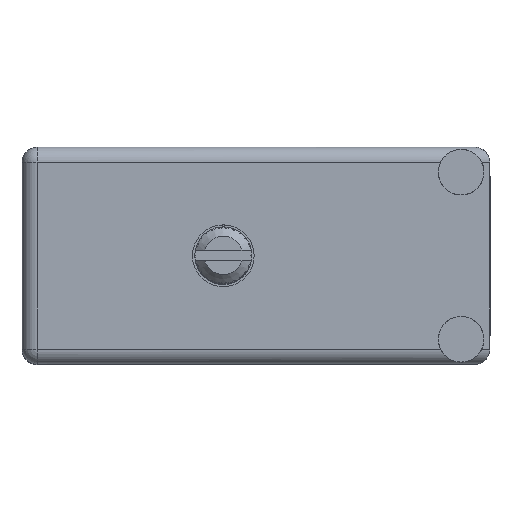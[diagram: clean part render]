
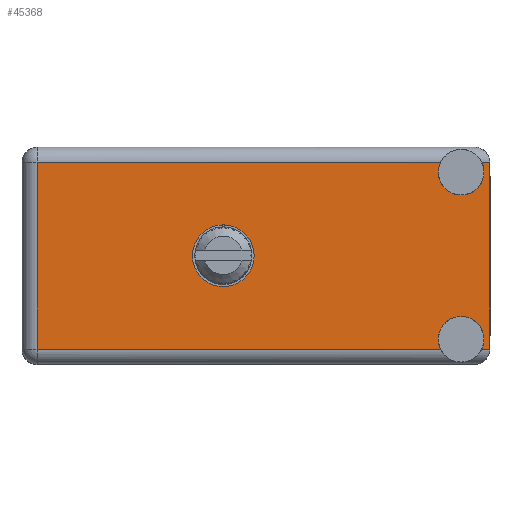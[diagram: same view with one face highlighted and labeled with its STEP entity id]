
A CAD part, top view. The second image highlights one B-rep face of the part: STEP entity #45368.
In plain terms, the highlighted face is planar.
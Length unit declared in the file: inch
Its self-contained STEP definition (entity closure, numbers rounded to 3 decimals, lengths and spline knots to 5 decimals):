
#1294 = VERTEX_POINT ( 'NONE', #162878 ) ;
#2491 = LINE ( 'NONE', #105582, #120860 ) ;
#3079 = EDGE_CURVE ( 'NONE', #1294, #177428, #159505, .T. ) ;
#6023 = ORIENTED_EDGE ( 'NONE', *, *, #139599, .F. ) ;
#8165 = EDGE_LOOP ( 'NONE', ( #48326, #6023, #74118, #162104, #158377, #182573, #144816, #176482, #103354, #86603 ) ) ;
#10953 = CARTESIAN_POINT ( 'NONE',  ( 1.445, 0.906, -0.1575 ) ) ;
#11195 = AXIS2_PLACEMENT_3D ( 'NONE', #15389, #90381, #115714 ) ;
#13502 = ORIENTED_EDGE ( 'NONE', *, *, #179214, .F. ) ;
#15389 = CARTESIAN_POINT ( 'NONE',  ( 1.445, 0.906, -0.6325 ) ) ;
#28520 = DIRECTION ( 'NONE',  ( 0., 0., 1. ) ) ;
#30066 = DIRECTION ( 'NONE',  ( -1., 0., 0. ) ) ;
#32092 = LINE ( 'NONE', #105170, #139621 ) ;
#32625 = DIRECTION ( 'NONE',  ( 1., 0., 0. ) ) ;
#34725 = VECTOR ( 'NONE', #75113, 39.37008 ) ;
#34835 = DIRECTION ( 'NONE',  ( 1., 0., 0. ) ) ;
#39893 = EDGE_CURVE ( 'NONE', #51134, #92540, #2491, .T. ) ;
#41580 = CIRCLE ( 'NONE', #113403, 0.075 ) ;
#43859 = DIRECTION ( 'NONE',  ( 0., 0., 1. ) ) ;
#45368 = ADVANCED_FACE ( 'NONE', ( #126077, #184150 ), #56694, .T. ) ;
#46123 = CARTESIAN_POINT ( 'NONE',  ( 1.445, 0.906, -0.0825 ) ) ;
#47203 = CIRCLE ( 'NONE', #163909, 0.1015 ) ;
#47387 = CARTESIAN_POINT ( 'NONE',  ( 0.6625, 0.906, -0.3575 ) ) ;
#47445 = ORIENTED_EDGE ( 'NONE', *, *, #75658, .F. ) ;
#48018 = DIRECTION ( 'NONE',  ( 0., 0., 1. ) ) ;
#48326 = ORIENTED_EDGE ( 'NONE', *, *, #91552, .T. ) ;
#49850 = DIRECTION ( 'NONE',  ( -1., 0., 0. ) ) ;
#49929 = CIRCLE ( 'NONE', #175555, 0.1015 ) ;
#51134 = VERTEX_POINT ( 'NONE', #149179 ) ;
#51189 = VERTEX_POINT ( 'NONE', #95678 ) ;
#56694 = PLANE ( 'NONE',  #162783 ) ;
#59122 = VERTEX_POINT ( 'NONE', #104556 ) ;
#59716 = DIRECTION ( 'NONE',  ( 0., 0., 1. ) ) ;
#60957 = CARTESIAN_POINT ( 'NONE',  ( 1.539, 0.906, -0.05 ) ) ;
#73524 = DIRECTION ( 'NONE',  ( 0., 0., 1. ) ) ;
#74118 = ORIENTED_EDGE ( 'NONE', *, *, #185371, .F. ) ;
#74225 = VERTEX_POINT ( 'NONE', #184911 ) ;
#74305 = EDGE_CURVE ( 'NONE', #51134, #59122, #32092, .T. ) ;
#75113 = DIRECTION ( 'NONE',  ( 0., 0., 1. ) ) ;
#75507 = DIRECTION ( 'NONE',  ( 0., 1., 0. ) ) ;
#75658 = EDGE_CURVE ( 'NONE', #74225, #164639, #49929, .T. ) ;
#76954 = VERTEX_POINT ( 'NONE', #10953 ) ;
#77851 = CARTESIAN_POINT ( 'NONE',  ( 0.6625, 0.906, -0.459 ) ) ;
#77945 = DIRECTION ( 'NONE',  ( 0., 0., 1. ) ) ;
#85773 = VECTOR ( 'NONE', #30066, 39.37008 ) ;
#86603 = ORIENTED_EDGE ( 'NONE', *, *, #3079, .T. ) ;
#90114 = CARTESIAN_POINT ( 'NONE',  ( 0.05, 0.906, -0.715 ) ) ;
#90381 = DIRECTION ( 'NONE',  ( 0., 1., 0. ) ) ;
#91552 = EDGE_CURVE ( 'NONE', #177428, #160019, #134212, .T. ) ;
#92540 = VERTEX_POINT ( 'NONE', #60957 ) ;
#95678 = CARTESIAN_POINT ( 'NONE',  ( 1.37741, 0.906, -0.665 ) ) ;
#96912 = CARTESIAN_POINT ( 'NONE',  ( 1.51259, 0.906, -0.05 ) ) ;
#97432 = CIRCLE ( 'NONE', #127371, 0.075 ) ;
#103145 = CARTESIAN_POINT ( 'NONE',  ( 0., 0.906, -0.665 ) ) ;
#103354 = ORIENTED_EDGE ( 'NONE', *, *, #135559, .T. ) ;
#104556 = CARTESIAN_POINT ( 'NONE',  ( 1.51259, 0.906, -0.665 ) ) ;
#105092 = CARTESIAN_POINT ( 'NONE',  ( 0.05, 0.906, -0.05 ) ) ;
#105170 = CARTESIAN_POINT ( 'NONE',  ( 0., 0.906, -0.665 ) ) ;
#105582 = CARTESIAN_POINT ( 'NONE',  ( 1.539, 0.906, 0. ) ) ;
#106069 = DIRECTION ( 'NONE',  ( 0., 1., 0. ) ) ;
#109537 = EDGE_LOOP ( 'NONE', ( #47445, #13502 ) ) ;
#113403 = AXIS2_PLACEMENT_3D ( 'NONE', #46123, #106069, #77945 ) ;
#115714 = DIRECTION ( 'NONE',  ( 0., 0., 1. ) ) ;
#119751 = LINE ( 'NONE', #178782, #157904 ) ;
#120860 = VECTOR ( 'NONE', #59716, 39.37008 ) ;
#121095 = DIRECTION ( 'NONE',  ( 0., 1., 0. ) ) ;
#125157 = CARTESIAN_POINT ( 'NONE',  ( 0., 0.906, -0.715 ) ) ;
#126077 = FACE_BOUND ( 'NONE', #109537, .T. ) ;
#126534 = CARTESIAN_POINT ( 'NONE',  ( 1.37741, 0.906, -0.05 ) ) ;
#127371 = AXIS2_PLACEMENT_3D ( 'NONE', #160689, #131636, #73524 ) ;
#131636 = DIRECTION ( 'NONE',  ( 0., 1., 0. ) ) ;
#134212 = LINE ( 'NONE', #163275, #153678 ) ;
#134365 = VERTEX_POINT ( 'NONE', #96912 ) ;
#134507 = EDGE_CURVE ( 'NONE', #51189, #141130, #156145, .T. ) ;
#135559 = EDGE_CURVE ( 'NONE', #51189, #1294, #172537, .T. ) ;
#137327 = DIRECTION ( 'NONE',  ( 0., 0., 1. ) ) ;
#139599 = EDGE_CURVE ( 'NONE', #76954, #160019, #97432, .T. ) ;
#139621 = VECTOR ( 'NONE', #49850, 39.37008 ) ;
#141130 = VERTEX_POINT ( 'NONE', #161004 ) ;
#144816 = ORIENTED_EDGE ( 'NONE', *, *, #171478, .F. ) ;
#149179 = CARTESIAN_POINT ( 'NONE',  ( 1.539, 0.906, -0.665 ) ) ;
#149661 = EDGE_CURVE ( 'NONE', #134365, #92540, #119751, .T. ) ;
#153678 = VECTOR ( 'NONE', #34835, 39.37008 ) ;
#156066 = DIRECTION ( 'NONE',  ( 0., 1., 0. ) ) ;
#156145 = CIRCLE ( 'NONE', #174043, 0.075 ) ;
#156401 = CARTESIAN_POINT ( 'NONE',  ( 0.6625, 0.906, -0.3575 ) ) ;
#157904 = VECTOR ( 'NONE', #32625, 39.37008 ) ;
#158377 = ORIENTED_EDGE ( 'NONE', *, *, #39893, .F. ) ;
#159505 = LINE ( 'NONE', #90114, #34725 ) ;
#160019 = VERTEX_POINT ( 'NONE', #126534 ) ;
#160551 = CIRCLE ( 'NONE', #11195, 0.075 ) ;
#160689 = CARTESIAN_POINT ( 'NONE',  ( 1.445, 0.906, -0.0825 ) ) ;
#161004 = CARTESIAN_POINT ( 'NONE',  ( 1.445, 0.906, -0.5575 ) ) ;
#162104 = ORIENTED_EDGE ( 'NONE', *, *, #149661, .T. ) ;
#162783 = AXIS2_PLACEMENT_3D ( 'NONE', #125157, #156066, #28520 ) ;
#162878 = CARTESIAN_POINT ( 'NONE',  ( 0.05, 0.906, -0.665 ) ) ;
#163275 = CARTESIAN_POINT ( 'NONE',  ( 1.539, 0.906, -0.05 ) ) ;
#163909 = AXIS2_PLACEMENT_3D ( 'NONE', #156401, #184475, #43859 ) ;
#164639 = VERTEX_POINT ( 'NONE', #77851 ) ;
#171478 = EDGE_CURVE ( 'NONE', #141130, #59122, #160551, .T. ) ;
#172537 = LINE ( 'NONE', #103145, #85773 ) ;
#174043 = AXIS2_PLACEMENT_3D ( 'NONE', #176423, #121095, #48018 ) ;
#175555 = AXIS2_PLACEMENT_3D ( 'NONE', #47387, #75507, #137327 ) ;
#176423 = CARTESIAN_POINT ( 'NONE',  ( 1.445, 0.906, -0.6325 ) ) ;
#176482 = ORIENTED_EDGE ( 'NONE', *, *, #134507, .F. ) ;
#177428 = VERTEX_POINT ( 'NONE', #105092 ) ;
#178782 = CARTESIAN_POINT ( 'NONE',  ( 1.539, 0.906, -0.05 ) ) ;
#179214 = EDGE_CURVE ( 'NONE', #164639, #74225, #47203, .T. ) ;
#182573 = ORIENTED_EDGE ( 'NONE', *, *, #74305, .T. ) ;
#184150 = FACE_OUTER_BOUND ( 'NONE', #8165, .T. ) ;
#184475 = DIRECTION ( 'NONE',  ( 0., 1., 0. ) ) ;
#184911 = CARTESIAN_POINT ( 'NONE',  ( 0.6625, 0.906, -0.256 ) ) ;
#185371 = EDGE_CURVE ( 'NONE', #134365, #76954, #41580, .T. ) ;
